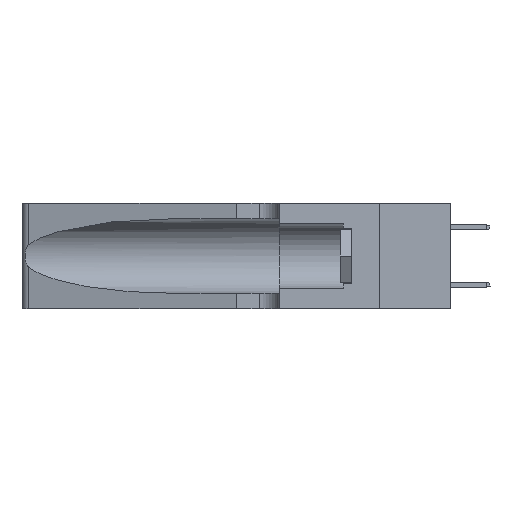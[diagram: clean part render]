
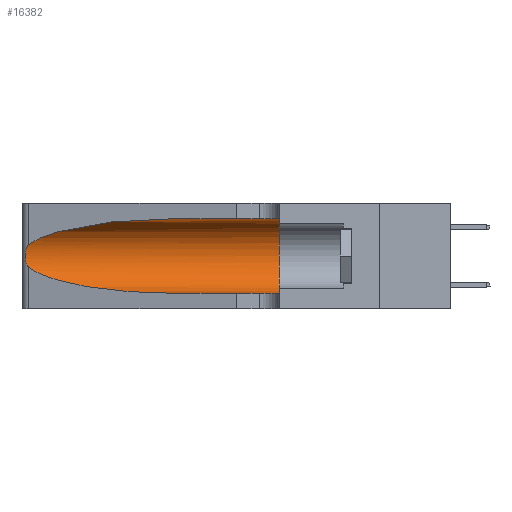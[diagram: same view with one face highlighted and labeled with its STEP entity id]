
A CAD part, left-side view. The second image highlights one B-rep face of the part: STEP entity #16382.
In plain terms, the highlighted cylindrical face has radius 3.308 mm (diameter 6.617 mm), a partial arc.
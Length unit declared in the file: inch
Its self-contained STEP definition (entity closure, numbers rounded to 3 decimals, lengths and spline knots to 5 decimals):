
#287 = CARTESIAN_POINT ( 'NONE',  ( 0.25789, 1.23486, 0.15765 ) ) ;
#1503 = ORIENTED_EDGE ( 'NONE', *, *, #9200, .T. ) ;
#1538 = CARTESIAN_POINT ( 'NONE',  ( 0.1305, 1.61858, 0.05475 ) ) ;
#1893 = CARTESIAN_POINT ( 'NONE',  ( 0.25856, 1.23593, 0.16098 ) ) ;
#1988 = EDGE_CURVE ( 'NONE', #11667, #17591, #17694, .T. ) ;
#2032 = VECTOR ( 'NONE', #12410, 39.37008 ) ;
#2141 = VECTOR ( 'NONE', #9368, 39.37008 ) ;
#2446 = DIRECTION ( 'NONE',  ( 0., 0., -1. ) ) ;
#2700 = CARTESIAN_POINT ( 'NONE',  ( 0.18966, 0.96281, 0.05475 ) ) ;
#4057 = CARTESIAN_POINT ( 'NONE',  ( 0.1305, 0.72297, 0.05475 ) ) ;
#4090 = CARTESIAN_POINT ( 'NONE',  ( 0.26075, 1.23896, 0.19203 ) ) ;
#4297 = DIRECTION ( 'NONE',  ( 0., -1., 0. ) ) ;
#4307 = VERTEX_POINT ( 'NONE', #10855 ) ;
#4709 = ORIENTED_EDGE ( 'NONE', *, *, #1988, .T. ) ;
#4792 = EDGE_CURVE ( 'NONE', #5063, #18917, #12531, .T. ) ;
#4903 = CARTESIAN_POINT ( 'NONE',  ( 0.25487, 1.22718, 0.14631 ) ) ;
#5063 = VERTEX_POINT ( 'NONE', #4903 ) ;
#5287 = CARTESIAN_POINT ( 'NONE',  ( 0.2373, 1.15595, 0.28018 ) ) ;
#5577 = CARTESIAN_POINT ( 'NONE',  ( 0.25787, 1.23484, 0.2124 ) ) ;
#5657 = EDGE_LOOP ( 'NONE', ( #4709, #18711, #19006, #1503, #17439, #15405 ) ) ;
#5944 = CARTESIAN_POINT ( 'NONE',  ( 0.25487, 1.22718, 0.14631 ) ) ;
#6143 = FACE_OUTER_BOUND ( 'NONE', #5657, .T. ) ;
#7023 = CARTESIAN_POINT ( 'NONE',  ( 0.18966, 0.96281, 0.31525 ) ) ;
#7298 = CARTESIAN_POINT ( 'NONE',  ( 0.25487, 1.22718, 0.22369 ) ) ;
#8217 = DIRECTION ( 'NONE',  ( 0., 0., 1. ) ) ;
#9082 = CARTESIAN_POINT ( 'NONE',  ( 0.25487, 1.22718, 0.22369 ) ) ;
#9200 = EDGE_CURVE ( 'NONE', #18917, #16342, #16363, .T. ) ;
#9270 = B_SPLINE_CURVE_WITH_KNOTS ( 'NONE', 3,
 ( #7298, #14740, #22214, #5577, #15106, #11052, #4090, #15236, #24152, #1893, #287, #11540, #20477, #5944 ),
 .UNSPECIFIED., .F., .F.,
 ( 4, 2, 2, 2, 2, 2, 4 ),
 ( 0., 0.00027, 0.00053, 0.00107, 0.0016, 0.00187, 0.00214 ),
 .UNSPECIFIED. ) ;
#9329 = EDGE_CURVE ( 'NONE', #17591, #5063, #9270, .T. ) ;
#9368 = DIRECTION ( 'NONE',  ( 0., -1., 0. ) ) ;
#10395 = CARTESIAN_POINT ( 'NONE',  ( 0.1305, 0.72297, 0.31525 ) ) ;
#10855 = CARTESIAN_POINT ( 'NONE',  ( 0.1305, 0.35, 0.31525 ) ) ;
#11052 = CARTESIAN_POINT ( 'NONE',  ( 0.26018, 1.23835, 0.19895 ) ) ;
#11282 = EDGE_CURVE ( 'NONE', #11667, #4307, #23903, .T. ) ;
#11487 = CARTESIAN_POINT ( 'NONE',  ( 0.1305, 0.35, 0.05475 ) ) ;
#11540 = CARTESIAN_POINT ( 'NONE',  ( 0.25639, 1.23186, 0.15144 ) ) ;
#11632 = CARTESIAN_POINT ( 'NONE',  ( 0.25487, 1.22718, 0.14631 ) ) ;
#11667 = VERTEX_POINT ( 'NONE', #10395 ) ;
#12410 = DIRECTION ( 'NONE',  ( 0., -1., 0. ) ) ;
#12531 =( BOUNDED_CURVE ( )  B_SPLINE_CURVE ( 3, ( #11632, #19334, #2700, #4057 ),
 .UNSPECIFIED., .F., .T. ) 
 B_SPLINE_CURVE_WITH_KNOTS ( ( 4, 4 ),
 ( 3.44316, 4.71239 ),
 .UNSPECIFIED. ) 
 CURVE ( )  GEOMETRIC_REPRESENTATION_ITEM ( )  RATIONAL_B_SPLINE_CURVE ( ( 1., 0.87, 0.87, 1. ) ) 
 REPRESENTATION_ITEM ( '' )  );
#12593 = CARTESIAN_POINT ( 'NONE',  ( 0.1305, 0.72297, 0.31525 ) ) ;
#13439 = CARTESIAN_POINT ( 'NONE',  ( 0.25487, 1.22718, 0.22369 ) ) ;
#13549 = AXIS2_PLACEMENT_3D ( 'NONE', #18972, #4297, #2446 ) ;
#13672 = DIRECTION ( 'NONE',  ( 0., 1., 0. ) ) ;
#14040 = CARTESIAN_POINT ( 'NONE',  ( 0.1305, 0.72297, 0.05475 ) ) ;
#14428 = AXIS2_PLACEMENT_3D ( 'NONE', #21625, #13672, #8217 ) ;
#14740 = CARTESIAN_POINT ( 'NONE',  ( 0.25555, 1.22994, 0.2215 ) ) ;
#15106 = CARTESIAN_POINT ( 'NONE',  ( 0.25854, 1.2359, 0.20912 ) ) ;
#15236 = CARTESIAN_POINT ( 'NONE',  ( 0.26075, 1.23896, 0.178 ) ) ;
#15405 = ORIENTED_EDGE ( 'NONE', *, *, #11282, .F. ) ;
#16342 = VERTEX_POINT ( 'NONE', #11487 ) ;
#16363 = LINE ( 'NONE', #1538, #2032 ) ;
#16382 = ADVANCED_FACE ( 'NONE', ( #6143 ), #21057, .F. ) ;
#17439 = ORIENTED_EDGE ( 'NONE', *, *, #20333, .F. ) ;
#17591 = VERTEX_POINT ( 'NONE', #13439 ) ;
#17694 =( BOUNDED_CURVE ( )  B_SPLINE_CURVE ( 3, ( #12593, #7023, #5287, #9082 ),
 .UNSPECIFIED., .F., .T. ) 
 B_SPLINE_CURVE_WITH_KNOTS ( ( 4, 4 ),
 ( 1.5708, 2.84003 ),
 .UNSPECIFIED. ) 
 CURVE ( )  GEOMETRIC_REPRESENTATION_ITEM ( )  RATIONAL_B_SPLINE_CURVE ( ( 1., 0.87, 0.87, 1. ) ) 
 REPRESENTATION_ITEM ( '' )  );
#18711 = ORIENTED_EDGE ( 'NONE', *, *, #9329, .T. ) ;
#18917 = VERTEX_POINT ( 'NONE', #14040 ) ;
#18972 = CARTESIAN_POINT ( 'NONE',  ( 0.1305, 1.61858, 0.185 ) ) ;
#19006 = ORIENTED_EDGE ( 'NONE', *, *, #4792, .T. ) ;
#19334 = CARTESIAN_POINT ( 'NONE',  ( 0.2373, 1.15595, 0.08982 ) ) ;
#20333 = EDGE_CURVE ( 'NONE', #4307, #16342, #21446, .T. ) ;
#20477 = CARTESIAN_POINT ( 'NONE',  ( 0.25555, 1.22993, 0.14849 ) ) ;
#21057 = CYLINDRICAL_SURFACE ( 'NONE', #13549, 0.13025 ) ;
#21446 = CIRCLE ( 'NONE', #14428, 0.13025 ) ;
#21625 = CARTESIAN_POINT ( 'NONE',  ( 0.1305, 0.35, 0.185 ) ) ;
#21962 = CARTESIAN_POINT ( 'NONE',  ( 0.1305, 1.61858, 0.31525 ) ) ;
#22214 = CARTESIAN_POINT ( 'NONE',  ( 0.25639, 1.23184, 0.21858 ) ) ;
#23903 = LINE ( 'NONE', #21962, #2141 ) ;
#24152 = CARTESIAN_POINT ( 'NONE',  ( 0.26017, 1.23833, 0.17102 ) ) ;
